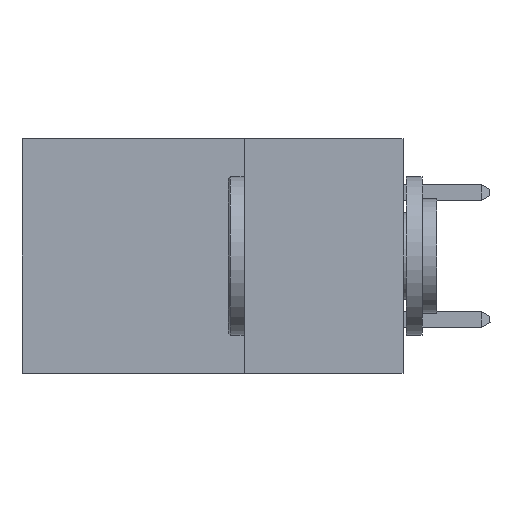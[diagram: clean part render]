
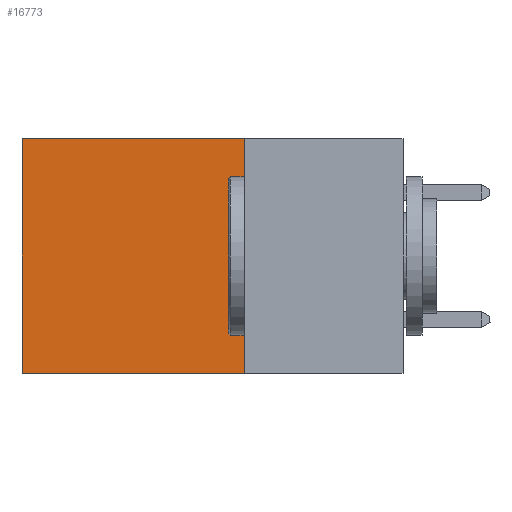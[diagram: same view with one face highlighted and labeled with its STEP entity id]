
A CAD part, left-side view. The second image highlights one B-rep face of the part: STEP entity #16773.
In plain terms, the highlighted planar face has unit normal (-1, 0, 0).
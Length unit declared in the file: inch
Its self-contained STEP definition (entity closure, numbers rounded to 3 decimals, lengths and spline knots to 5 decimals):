
#313 = LINE ( 'NONE', #22709, #16149 ) ;
#480 = EDGE_LOOP ( 'NONE', ( #23943, #3874, #14929, #39398 ) ) ;
#3874 = ORIENTED_EDGE ( 'NONE', *, *, #37373, .F. ) ;
#4183 = DIRECTION ( 'NONE',  ( 0., 0., -1. ) ) ;
#5922 = CARTESIAN_POINT ( 'NONE',  ( 0.2875, 0.25, 0. ) ) ;
#10895 = VECTOR ( 'NONE', #37531, 39.37008 ) ;
#12141 = VERTEX_POINT ( 'NONE', #38355 ) ;
#12994 = DIRECTION ( 'NONE',  ( 0., 1., 0. ) ) ;
#14319 = VECTOR ( 'NONE', #4183, 39.37008 ) ;
#14929 = ORIENTED_EDGE ( 'NONE', *, *, #25008, .F. ) ;
#15851 = EDGE_CURVE ( 'NONE', #12141, #36686, #313, .T. ) ;
#15931 = VECTOR ( 'NONE', #17060, 39.37008 ) ;
#16149 = VECTOR ( 'NONE', #12994, 39.37008 ) ;
#16773 = ADVANCED_FACE ( 'NONE', ( #36167 ), #33984, .F. ) ;
#17060 = DIRECTION ( 'NONE',  ( 0., 0., -1. ) ) ;
#21777 = CARTESIAN_POINT ( 'NONE',  ( 0.2875, 0.6, -0.37 ) ) ;
#22709 = CARTESIAN_POINT ( 'NONE',  ( 0.2875, 0.25, 0. ) ) ;
#23310 = CARTESIAN_POINT ( 'NONE',  ( 0.2875, 0.25, 0. ) ) ;
#23943 = ORIENTED_EDGE ( 'NONE', *, *, #36236, .T. ) ;
#24653 = DIRECTION ( 'NONE',  ( 0., 0., -1. ) ) ;
#24830 = VERTEX_POINT ( 'NONE', #28928 ) ;
#25008 = EDGE_CURVE ( 'NONE', #12141, #24830, #36535, .T. ) ;
#27067 = VERTEX_POINT ( 'NONE', #21777 ) ;
#27200 = LINE ( 'NONE', #29085, #14319 ) ;
#28928 = CARTESIAN_POINT ( 'NONE',  ( 0.2875, 0.25, -0.37 ) ) ;
#29085 = CARTESIAN_POINT ( 'NONE',  ( 0.2875, 0.6, 0. ) ) ;
#31177 = CARTESIAN_POINT ( 'NONE',  ( 0.2875, 0.25, -0.37 ) ) ;
#33984 = PLANE ( 'NONE',  #34371 ) ;
#34371 = AXIS2_PLACEMENT_3D ( 'NONE', #5922, #36897, #24653 ) ;
#34677 = CARTESIAN_POINT ( 'NONE',  ( 0.2875, 0.6, 0. ) ) ;
#36167 = FACE_OUTER_BOUND ( 'NONE', #480, .T. ) ;
#36236 = EDGE_CURVE ( 'NONE', #36686, #27067, #27200, .T. ) ;
#36391 = LINE ( 'NONE', #31177, #10895 ) ;
#36535 = LINE ( 'NONE', #23310, #15931 ) ;
#36686 = VERTEX_POINT ( 'NONE', #34677 ) ;
#36897 = DIRECTION ( 'NONE',  ( 1., 0., 0. ) ) ;
#37373 = EDGE_CURVE ( 'NONE', #24830, #27067, #36391, .T. ) ;
#37531 = DIRECTION ( 'NONE',  ( 0., 1., 0. ) ) ;
#38355 = CARTESIAN_POINT ( 'NONE',  ( 0.2875, 0.25, 0. ) ) ;
#39398 = ORIENTED_EDGE ( 'NONE', *, *, #15851, .T. ) ;
